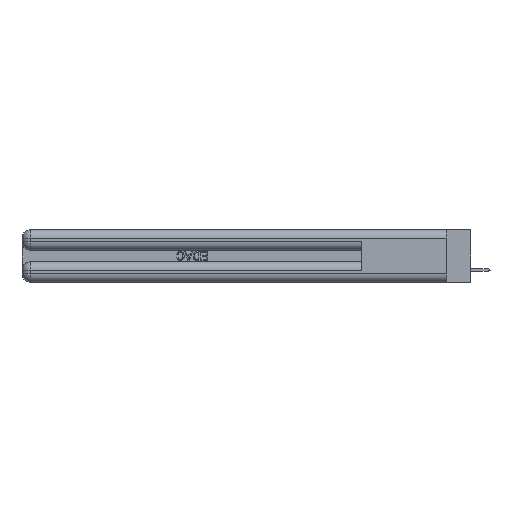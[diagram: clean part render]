
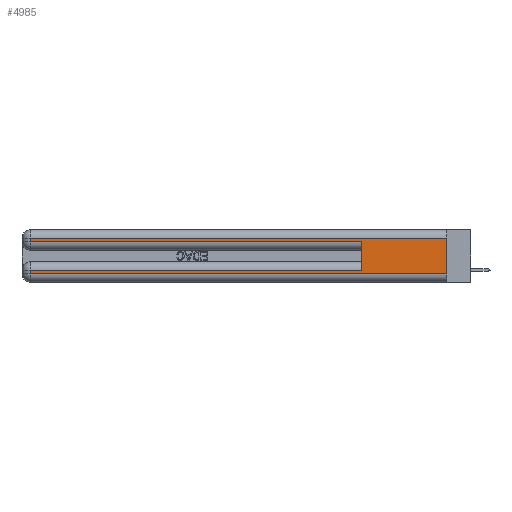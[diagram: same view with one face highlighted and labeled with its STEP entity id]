
A CAD part, left-side view. The second image highlights one B-rep face of the part: STEP entity #4985.
In plain terms, the highlighted planar face has unit normal (-1, 0, 0).
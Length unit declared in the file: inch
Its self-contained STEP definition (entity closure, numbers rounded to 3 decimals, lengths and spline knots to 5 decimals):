
#124 = VECTOR ( 'NONE', #19210, 39.37008 ) ;
#487 = EDGE_LOOP ( 'NONE', ( #23401, #22829, #35925, #924, #9242, #31323, #35940, #24652 ) ) ;
#700 = DIRECTION ( 'NONE',  ( 0., 0., 1. ) ) ;
#862 = VECTOR ( 'NONE', #33983, 39.37008 ) ;
#924 = ORIENTED_EDGE ( 'NONE', *, *, #8441, .T. ) ;
#1766 = DIRECTION ( 'NONE',  ( 0., 0., -1. ) ) ;
#2825 = VERTEX_POINT ( 'NONE', #12864 ) ;
#3283 = EDGE_CURVE ( 'NONE', #21220, #30481, #6478, .T. ) ;
#3504 = LINE ( 'NONE', #14747, #18667 ) ;
#4170 = CARTESIAN_POINT ( 'NONE',  ( 0., 0., 0.06 ) ) ;
#4358 = DIRECTION ( 'NONE',  ( 0., -1., 0. ) ) ;
#4832 = VECTOR ( 'NONE', #24116, 39.37008 ) ;
#4985 = ADVANCED_FACE ( 'NONE', ( #32468 ), #6818, .F. ) ;
#6478 = LINE ( 'NONE', #16011, #29953 ) ;
#6661 = VERTEX_POINT ( 'NONE', #14079 ) ;
#6818 = PLANE ( 'NONE',  #29937 ) ;
#7165 = CARTESIAN_POINT ( 'NONE',  ( 0., 0., 0.37 ) ) ;
#7361 = DIRECTION ( 'NONE',  ( 1., 0., 0. ) ) ;
#7625 = DIRECTION ( 'NONE',  ( 0., -1., 0. ) ) ;
#7777 = CARTESIAN_POINT ( 'NONE',  ( 0., 0., 0.37 ) ) ;
#8441 = EDGE_CURVE ( 'NONE', #30481, #6661, #32909, .T. ) ;
#9242 = ORIENTED_EDGE ( 'NONE', *, *, #17716, .F. ) ;
#9368 = CARTESIAN_POINT ( 'NONE',  ( 0., 0.6, 0.085 ) ) ;
#9801 = VECTOR ( 'NONE', #26446, 39.37008 ) ;
#10886 = VECTOR ( 'NONE', #7625, 39.37008 ) ;
#11247 = EDGE_CURVE ( 'NONE', #19814, #21220, #33602, .T. ) ;
#12000 = CARTESIAN_POINT ( 'NONE',  ( 0., 2.94, 0.37 ) ) ;
#12864 = CARTESIAN_POINT ( 'NONE',  ( 0., 2.94, 0.06 ) ) ;
#13155 = VERTEX_POINT ( 'NONE', #22898 ) ;
#13935 = CARTESIAN_POINT ( 'NONE',  ( 0., 0., 0.31 ) ) ;
#14079 = CARTESIAN_POINT ( 'NONE',  ( 0., 0.6, 0.285 ) ) ;
#14747 = CARTESIAN_POINT ( 'NONE',  ( 0., 0.6, 0.145 ) ) ;
#16011 = CARTESIAN_POINT ( 'NONE',  ( 0., 2.94, 0.37 ) ) ;
#16562 = EDGE_CURVE ( 'NONE', #35008, #18067, #32725, .T. ) ;
#17716 = EDGE_CURVE ( 'NONE', #35008, #6661, #3504, .T. ) ;
#18067 = VERTEX_POINT ( 'NONE', #26315 ) ;
#18667 = VECTOR ( 'NONE', #700, 39.37008 ) ;
#18675 = CARTESIAN_POINT ( 'NONE',  ( 0., 0., 0.085 ) ) ;
#18795 = DIRECTION ( 'NONE',  ( 0., 0., -1. ) ) ;
#19210 = DIRECTION ( 'NONE',  ( 0., 0., -1. ) ) ;
#19814 = VERTEX_POINT ( 'NONE', #24795 ) ;
#19841 = EDGE_CURVE ( 'NONE', #2825, #13155, #36024, .T. ) ;
#20460 = CARTESIAN_POINT ( 'NONE',  ( 0., 2.94, 0.31 ) ) ;
#21220 = VERTEX_POINT ( 'NONE', #20460 ) ;
#21259 = EDGE_CURVE ( 'NONE', #18067, #2825, #31685, .T. ) ;
#22829 = ORIENTED_EDGE ( 'NONE', *, *, #11247, .T. ) ;
#22898 = CARTESIAN_POINT ( 'NONE',  ( 0., 0., 0.06 ) ) ;
#23401 = ORIENTED_EDGE ( 'NONE', *, *, #30407, .F. ) ;
#24116 = DIRECTION ( 'NONE',  ( 0., 1., 0. ) ) ;
#24224 = CARTESIAN_POINT ( 'NONE',  ( 0., 2.94, 0.285 ) ) ;
#24652 = ORIENTED_EDGE ( 'NONE', *, *, #19841, .T. ) ;
#24795 = CARTESIAN_POINT ( 'NONE',  ( 0., 0., 0.31 ) ) ;
#25405 = LINE ( 'NONE', #7777, #124 ) ;
#26315 = CARTESIAN_POINT ( 'NONE',  ( 0., 2.94, 0.085 ) ) ;
#26446 = DIRECTION ( 'NONE',  ( 0., 0., -1. ) ) ;
#29937 = AXIS2_PLACEMENT_3D ( 'NONE', #7165, #7361, #18795 ) ;
#29953 = VECTOR ( 'NONE', #1766, 39.37008 ) ;
#30407 = EDGE_CURVE ( 'NONE', #19814, #13155, #25405, .T. ) ;
#30481 = VERTEX_POINT ( 'NONE', #24224 ) ;
#31323 = ORIENTED_EDGE ( 'NONE', *, *, #16562, .T. ) ;
#31685 = LINE ( 'NONE', #12000, #9801 ) ;
#32468 = FACE_OUTER_BOUND ( 'NONE', #487, .T. ) ;
#32725 = LINE ( 'NONE', #18675, #4832 ) ;
#32738 = CARTESIAN_POINT ( 'NONE',  ( 0., 0., 0.285 ) ) ;
#32909 = LINE ( 'NONE', #32738, #10886 ) ;
#33602 = LINE ( 'NONE', #13935, #862 ) ;
#33983 = DIRECTION ( 'NONE',  ( 0., 1., 0. ) ) ;
#35008 = VERTEX_POINT ( 'NONE', #9368 ) ;
#35058 = VECTOR ( 'NONE', #4358, 39.37008 ) ;
#35925 = ORIENTED_EDGE ( 'NONE', *, *, #3283, .T. ) ;
#35940 = ORIENTED_EDGE ( 'NONE', *, *, #21259, .T. ) ;
#36024 = LINE ( 'NONE', #4170, #35058 ) ;
